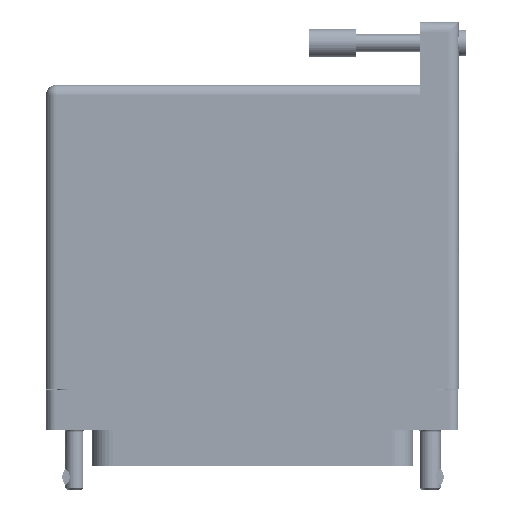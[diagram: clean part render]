
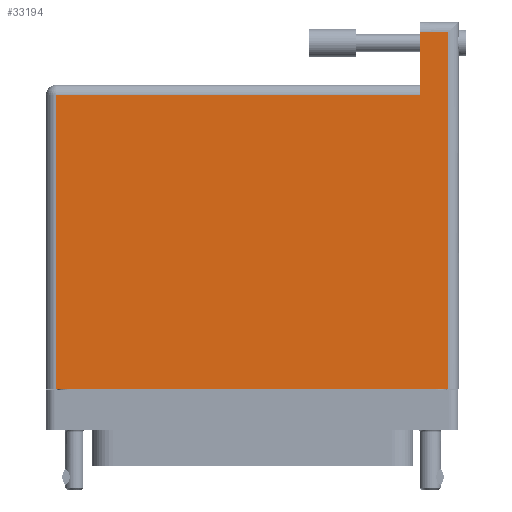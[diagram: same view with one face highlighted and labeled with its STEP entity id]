
A CAD part, front view. The second image highlights one B-rep face of the part: STEP entity #33194.
In plain terms, the highlighted face is planar.
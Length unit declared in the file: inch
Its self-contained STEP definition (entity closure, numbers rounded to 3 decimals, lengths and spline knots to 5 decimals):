
#2015 = DIRECTION ( 'NONE',  ( 1., 0., 0. ) ) ;
#5206 = EDGE_CURVE ( 'NONE', #84515, #93300, #6401, .T. ) ;
#5459 = ORIENTED_EDGE ( 'NONE', *, *, #28926, .T. ) ;
#6116 = LINE ( 'NONE', #89063, #8579 ) ;
#6401 = LINE ( 'NONE', #63141, #68454 ) ;
#6901 = LINE ( 'NONE', #55321, #97577 ) ;
#8579 = VECTOR ( 'NONE', #2015, 39.37008 ) ;
#8733 = VERTEX_POINT ( 'NONE', #88724 ) ;
#16585 = CARTESIAN_POINT ( 'NONE',  ( -1.3075, -0.1, 0.765 ) ) ;
#18422 = LINE ( 'NONE', #98676, #58155 ) ;
#21983 = VERTEX_POINT ( 'NONE', #98031 ) ;
#28926 = EDGE_CURVE ( 'NONE', #21983, #37908, #76830, .T. ) ;
#29311 = LINE ( 'NONE', #16585, #37957 ) ;
#30655 = DIRECTION ( 'NONE',  ( 0., 0., -1. ) ) ;
#32316 = CARTESIAN_POINT ( 'NONE',  ( 1.1215, 1.86, 0.765 ) ) ;
#33194 = ADVANCED_FACE ( 'NONE', ( #54629 ), #46294, .F. ) ;
#33805 = EDGE_CURVE ( 'NONE', #8733, #84515, #6116, .T. ) ;
#37908 = VERTEX_POINT ( 'NONE', #32316 ) ;
#37957 = VECTOR ( 'NONE', #48539, 39.37008 ) ;
#41451 = AXIS2_PLACEMENT_3D ( 'NONE', #93508, #30655, #70581 ) ;
#46294 = PLANE ( 'NONE',  #41451 ) ;
#47538 = EDGE_CURVE ( 'NONE', #93300, #21983, #6901, .T. ) ;
#48075 = DIRECTION ( 'NONE',  ( 0., -1., 0. ) ) ;
#48539 = DIRECTION ( 'NONE',  ( 0., -1., 0. ) ) ;
#51217 = DIRECTION ( 'NONE',  ( 0., 1., 0. ) ) ;
#54295 = ORIENTED_EDGE ( 'NONE', *, *, #47538, .T. ) ;
#54629 = FACE_OUTER_BOUND ( 'NONE', #101947, .T. ) ;
#55321 = CARTESIAN_POINT ( 'NONE',  ( -1.3775, 2.28, 0.765 ) ) ;
#55725 = VECTOR ( 'NONE', #48075, 39.37008 ) ;
#58155 = VECTOR ( 'NONE', #98318, 39.37008 ) ;
#63141 = CARTESIAN_POINT ( 'NONE',  ( 1.3075, 2.35, 0.765 ) ) ;
#65656 = DIRECTION ( 'NONE',  ( -1., 0., 0. ) ) ;
#67962 = EDGE_CURVE ( 'NONE', #37908, #80732, #18422, .T. ) ;
#68454 = VECTOR ( 'NONE', #51217, 39.37008 ) ;
#69490 = ORIENTED_EDGE ( 'NONE', *, *, #33805, .T. ) ;
#70581 = DIRECTION ( 'NONE',  ( -1., 0., 0. ) ) ;
#72430 = ORIENTED_EDGE ( 'NONE', *, *, #90792, .T. ) ;
#76830 = LINE ( 'NONE', #83876, #55725 ) ;
#80090 = CARTESIAN_POINT ( 'NONE',  ( -1.3075, 1.86, 0.765 ) ) ;
#80732 = VERTEX_POINT ( 'NONE', #80090 ) ;
#81305 = CARTESIAN_POINT ( 'NONE',  ( 1.3075, -0.1, 0.765 ) ) ;
#83876 = CARTESIAN_POINT ( 'NONE',  ( 1.1215, 2.35, 0.765 ) ) ;
#84515 = VERTEX_POINT ( 'NONE', #81305 ) ;
#88724 = CARTESIAN_POINT ( 'NONE',  ( -1.3075, -0.1, 0.765 ) ) ;
#89063 = CARTESIAN_POINT ( 'NONE',  ( -1.3775, -0.1, 0.765 ) ) ;
#90792 = EDGE_CURVE ( 'NONE', #80732, #8733, #29311, .T. ) ;
#91946 = ORIENTED_EDGE ( 'NONE', *, *, #67962, .T. ) ;
#93300 = VERTEX_POINT ( 'NONE', #96269 ) ;
#93508 = CARTESIAN_POINT ( 'NONE',  ( -1.3775, 1.93, 0.765 ) ) ;
#96269 = CARTESIAN_POINT ( 'NONE',  ( 1.3075, 2.28, 0.765 ) ) ;
#97577 = VECTOR ( 'NONE', #65656, 39.37008 ) ;
#98031 = CARTESIAN_POINT ( 'NONE',  ( 1.1215, 2.28, 0.765 ) ) ;
#98318 = DIRECTION ( 'NONE',  ( -1., 0., 0. ) ) ;
#98401 = ORIENTED_EDGE ( 'NONE', *, *, #5206, .T. ) ;
#98676 = CARTESIAN_POINT ( 'NONE',  ( -1.3775, 1.86, 0.765 ) ) ;
#101947 = EDGE_LOOP ( 'NONE', ( #5459, #91946, #72430, #69490, #98401, #54295 ) ) ;
